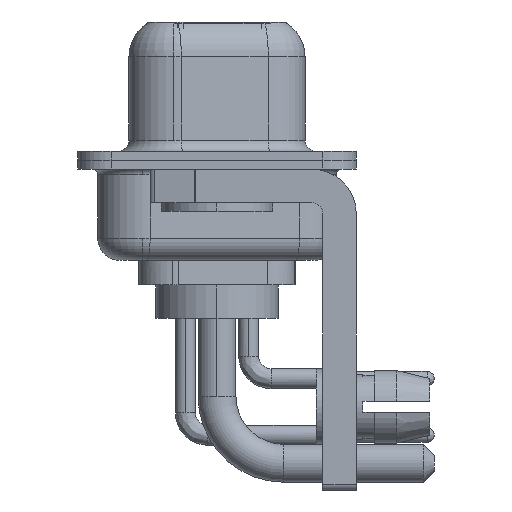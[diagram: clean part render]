
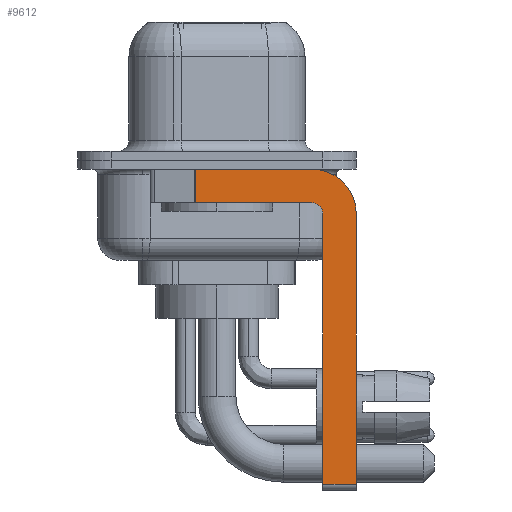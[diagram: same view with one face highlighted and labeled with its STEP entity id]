
A CAD part, left-side view. The second image highlights one B-rep face of the part: STEP entity #9612.
In plain terms, the highlighted planar face has unit normal (-1, 0, 0).
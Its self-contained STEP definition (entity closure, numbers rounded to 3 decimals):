
#290 = LINE ( 'NONE', #10684, #3560 ) ;
#559 = ORIENTED_EDGE ( 'NONE', *, *, #17274, .F. ) ;
#670 = AXIS2_PLACEMENT_3D ( 'NONE', #20628, #12260, #17298 ) ;
#905 = LINE ( 'NONE', #9585, #11597 ) ;
#1180 = ORIENTED_EDGE ( 'NONE', *, *, #21677, .F. ) ;
#1325 = CIRCLE ( 'NONE', #15544, 0.5 ) ;
#1432 = DIRECTION ( 'NONE',  ( 0., 0., -1. ) ) ;
#1691 = EDGE_CURVE ( 'NONE', #13157, #3382, #1800, .T. ) ;
#1800 = LINE ( 'NONE', #8766, #20822 ) ;
#1815 = ORIENTED_EDGE ( 'NONE', *, *, #9579, .F. ) ;
#2212 = EDGE_LOOP ( 'NONE', ( #559, #3585, #1180, #21219, #19413, #12475, #1815, #3936 ) ) ;
#2332 = DIRECTION ( 'NONE',  ( 0., 0., 1. ) ) ;
#2451 = DIRECTION ( 'NONE',  ( -1., 0., 0. ) ) ;
#3382 = VERTEX_POINT ( 'NONE', #15765 ) ;
#3560 = VECTOR ( 'NONE', #5440, 1000. ) ;
#3585 = ORIENTED_EDGE ( 'NONE', *, *, #1691, .T. ) ;
#3602 = VERTEX_POINT ( 'NONE', #13244 ) ;
#3936 = ORIENTED_EDGE ( 'NONE', *, *, #10388, .F. ) ;
#4414 = CARTESIAN_POINT ( 'NONE',  ( -2.9, -6.25, -14.55 ) ) ;
#5414 = VERTEX_POINT ( 'NONE', #10935 ) ;
#5440 = DIRECTION ( 'NONE',  ( 0., 0., 1. ) ) ;
#6917 = EDGE_CURVE ( 'NONE', #5414, #15756, #290, .T. ) ;
#7873 = DIRECTION ( 'NONE',  ( 0., -1., 0. ) ) ;
#8535 = VERTEX_POINT ( 'NONE', #13480 ) ;
#8766 = CARTESIAN_POINT ( 'NONE',  ( -2.9, 0.978, -1.9 ) ) ;
#9579 = EDGE_CURVE ( 'NONE', #8535, #21817, #19033, .T. ) ;
#9585 = CARTESIAN_POINT ( 'NONE',  ( -2.9, -4.25, -14.55 ) ) ;
#9612 = ADVANCED_FACE ( 'NONE', ( #13642 ), #20855, .F. ) ;
#10213 = EDGE_CURVE ( 'NONE', #15756, #18893, #1325, .T. ) ;
#10388 = EDGE_CURVE ( 'NONE', #3602, #8535, #15770, .T. ) ;
#10684 = CARTESIAN_POINT ( 'NONE',  ( -2.9, -4.75, -14.8 ) ) ;
#10772 = CARTESIAN_POINT ( 'NONE',  ( -2.9, -4.25, -2.4 ) ) ;
#10935 = CARTESIAN_POINT ( 'NONE',  ( -2.9, -4.75, -14.55 ) ) ;
#11128 = DIRECTION ( 'NONE',  ( 0., 1., 0. ) ) ;
#11597 = VECTOR ( 'NONE', #7873, 1000. ) ;
#12155 = DIRECTION ( 'NONE',  ( 0., -1., 0. ) ) ;
#12260 = DIRECTION ( 'NONE',  ( 1., 0., 0. ) ) ;
#12475 = ORIENTED_EDGE ( 'NONE', *, *, #19435, .T. ) ;
#12698 = VECTOR ( 'NONE', #1432, 1000. ) ;
#12844 = AXIS2_PLACEMENT_3D ( 'NONE', #22110, #21761, #18669 ) ;
#13157 = VERTEX_POINT ( 'NONE', #19186 ) ;
#13244 = CARTESIAN_POINT ( 'NONE',  ( -2.9, -4.25, -0.4 ) ) ;
#13480 = CARTESIAN_POINT ( 'NONE',  ( -2.9, -6.25, -2.4 ) ) ;
#13642 = FACE_OUTER_BOUND ( 'NONE', #2212, .T. ) ;
#13725 = CARTESIAN_POINT ( 'NONE',  ( -2.9, -4.75, -2.4 ) ) ;
#14254 = VECTOR ( 'NONE', #11128, 1000. ) ;
#14769 = CARTESIAN_POINT ( 'NONE',  ( -2.9, -4.25, -1.9 ) ) ;
#15368 = LINE ( 'NONE', #20753, #22567 ) ;
#15544 = AXIS2_PLACEMENT_3D ( 'NONE', #10772, #2451, #2332 ) ;
#15756 = VERTEX_POINT ( 'NONE', #13725 ) ;
#15765 = CARTESIAN_POINT ( 'NONE',  ( -2.9, 0.978, -1.9 ) ) ;
#15770 = CIRCLE ( 'NONE', #12844, 2. ) ;
#16964 = CARTESIAN_POINT ( 'NONE',  ( -2.9, -6.25, -2.4 ) ) ;
#17274 = EDGE_CURVE ( 'NONE', #13157, #3602, #15368, .T. ) ;
#17298 = DIRECTION ( 'NONE',  ( 0., 0., -1. ) ) ;
#17640 = CARTESIAN_POINT ( 'NONE',  ( -2.9, -4.25, -1.9 ) ) ;
#18224 = LINE ( 'NONE', #14769, #14254 ) ;
#18669 = DIRECTION ( 'NONE',  ( 0., 0., -1. ) ) ;
#18893 = VERTEX_POINT ( 'NONE', #17640 ) ;
#19033 = LINE ( 'NONE', #16964, #12698 ) ;
#19186 = CARTESIAN_POINT ( 'NONE',  ( -2.9, 0.978, -0.4 ) ) ;
#19413 = ORIENTED_EDGE ( 'NONE', *, *, #6917, .F. ) ;
#19435 = EDGE_CURVE ( 'NONE', #5414, #21817, #905, .T. ) ;
#19446 = DIRECTION ( 'NONE',  ( 0., 0., -1. ) ) ;
#20628 = CARTESIAN_POINT ( 'NONE',  ( -2.9, -4.25, -2.4 ) ) ;
#20753 = CARTESIAN_POINT ( 'NONE',  ( -2.9, 3., -0.4 ) ) ;
#20822 = VECTOR ( 'NONE', #19446, 1000. ) ;
#20855 = PLANE ( 'NONE',  #670 ) ;
#21219 = ORIENTED_EDGE ( 'NONE', *, *, #10213, .F. ) ;
#21677 = EDGE_CURVE ( 'NONE', #18893, #3382, #18224, .T. ) ;
#21761 = DIRECTION ( 'NONE',  ( 1., 0., 0. ) ) ;
#21817 = VERTEX_POINT ( 'NONE', #4414 ) ;
#22110 = CARTESIAN_POINT ( 'NONE',  ( -2.9, -4.25, -2.4 ) ) ;
#22567 = VECTOR ( 'NONE', #12155, 1000. ) ;
